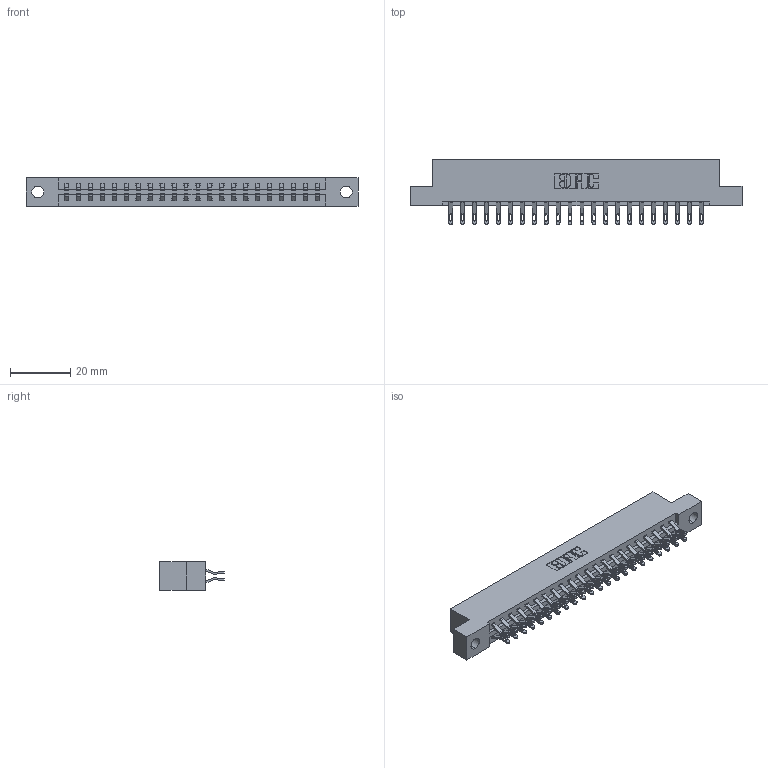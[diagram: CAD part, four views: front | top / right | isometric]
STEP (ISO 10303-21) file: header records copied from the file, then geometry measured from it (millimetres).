
FILE_DESCRIPTION (( 'STEP AP203' ), '1' );
FILE_NAME ('387-044-555-204.STEP', '2019-10-18T06:09:47', ( '' ), ( '' ), 'SwSTEP 2.0', 'SolidWorks 2016', '' );
FILE_SCHEMA (( 'CONFIG_CONTROL_DESIGN' ));
Length unit declared in the file: inch
Products named in the file (3): 387-044-555-204; 337 Part_Flush Mounting Lugs - 0.156 Dia-TH; 345-292-001_555 Tail
Assembly tree (45 placements, depth 2):
  387-044-555-204
    337 Part_Flush Mounting Lugs - 0.156 Dia-TH
    345-292-001_555 Tail  x44
Bounding box: 110.19 x 21.47 x 9.4 mm (x, y, z)
Volume: 11385.7 mm3; surface area: 12955.7 mm2
Topology: 45 solids, 45 shells, 2754 faces, 8627 edges, 5750 vertices
Faces by surface type: plane 1654, cylinder 1100
Entity records: 19973 total; most frequent: CARTESIAN_POINT 3416, ORIENTED_EDGE 3322, DIRECTION 2913, EDGE_CURVE 1661, VECTOR 1513, LINE 1513, VERTEX_POINT 1106, AXIS2_PLACEMENT_3D 700
